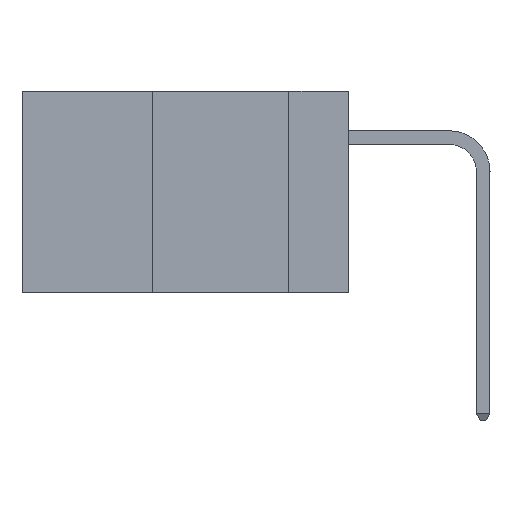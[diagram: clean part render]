
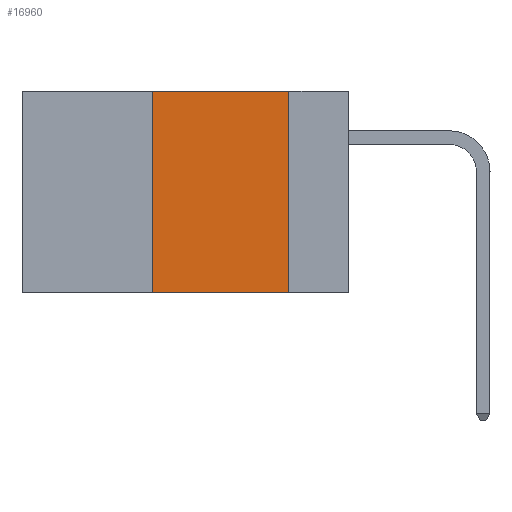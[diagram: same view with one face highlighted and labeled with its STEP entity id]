
A CAD part, left-side view. The second image highlights one B-rep face of the part: STEP entity #16960.
In plain terms, the highlighted planar face has unit normal (-1, 0, 0).
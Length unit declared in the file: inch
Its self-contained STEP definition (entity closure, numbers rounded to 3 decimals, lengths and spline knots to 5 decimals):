
#1099 = VECTOR ( 'NONE', #11082, 39.37008 ) ;
#1627 = DIRECTION ( 'NONE',  ( 0., -1., 0. ) ) ;
#2027 = CARTESIAN_POINT ( 'NONE',  ( 0., 0.36, 0. ) ) ;
#3140 = DIRECTION ( 'NONE',  ( 1., 0., 0. ) ) ;
#3811 = VERTEX_POINT ( 'NONE', #35199 ) ;
#4220 = ORIENTED_EDGE ( 'NONE', *, *, #22914, .F. ) ;
#4672 = EDGE_LOOP ( 'NONE', ( #24133, #18451, #4220, #6389 ) ) ;
#4808 = VECTOR ( 'NONE', #13511, 39.37008 ) ;
#6389 = ORIENTED_EDGE ( 'NONE', *, *, #15403, .T. ) ;
#7923 = VERTEX_POINT ( 'NONE', #24245 ) ;
#8269 = CARTESIAN_POINT ( 'NONE',  ( 0., 0.11, 0. ) ) ;
#8831 = FACE_OUTER_BOUND ( 'NONE', #4672, .T. ) ;
#9212 = LINE ( 'NONE', #18640, #10092 ) ;
#10092 = VECTOR ( 'NONE', #1627, 39.37008 ) ;
#11082 = DIRECTION ( 'NONE',  ( 0., 0., -1. ) ) ;
#12432 = LINE ( 'NONE', #2027, #4808 ) ;
#13511 = DIRECTION ( 'NONE',  ( 0., 0., 1. ) ) ;
#15403 = EDGE_CURVE ( 'NONE', #24219, #3811, #9212, .T. ) ;
#16215 = LINE ( 'NONE', #8269, #1099 ) ;
#16960 = ADVANCED_FACE ( 'NONE', ( #8831 ), #33936, .F. ) ;
#18451 = ORIENTED_EDGE ( 'NONE', *, *, #20109, .F. ) ;
#18640 = CARTESIAN_POINT ( 'NONE',  ( 0., 0.6, -0.37 ) ) ;
#19044 = VERTEX_POINT ( 'NONE', #34357 ) ;
#19118 = VECTOR ( 'NONE', #22319, 39.37008 ) ;
#19626 = CARTESIAN_POINT ( 'NONE',  ( 0., 0.6, 0. ) ) ;
#20079 = CARTESIAN_POINT ( 'NONE',  ( 0., 0.6, 0. ) ) ;
#20109 = EDGE_CURVE ( 'NONE', #7923, #19044, #33865, .T. ) ;
#22319 = DIRECTION ( 'NONE',  ( 0., -1., 0. ) ) ;
#22911 = DIRECTION ( 'NONE',  ( 0., 0., -1. ) ) ;
#22914 = EDGE_CURVE ( 'NONE', #24219, #7923, #12432, .T. ) ;
#24133 = ORIENTED_EDGE ( 'NONE', *, *, #24814, .F. ) ;
#24219 = VERTEX_POINT ( 'NONE', #28139 ) ;
#24245 = CARTESIAN_POINT ( 'NONE',  ( 0., 0.36, 0. ) ) ;
#24814 = EDGE_CURVE ( 'NONE', #19044, #3811, #16215, .T. ) ;
#26151 = AXIS2_PLACEMENT_3D ( 'NONE', #20079, #3140, #22911 ) ;
#28139 = CARTESIAN_POINT ( 'NONE',  ( 0., 0.36, -0.37 ) ) ;
#33865 = LINE ( 'NONE', #19626, #19118 ) ;
#33936 = PLANE ( 'NONE',  #26151 ) ;
#34357 = CARTESIAN_POINT ( 'NONE',  ( 0., 0.11, 0. ) ) ;
#35199 = CARTESIAN_POINT ( 'NONE',  ( 0., 0.11, -0.37 ) ) ;
